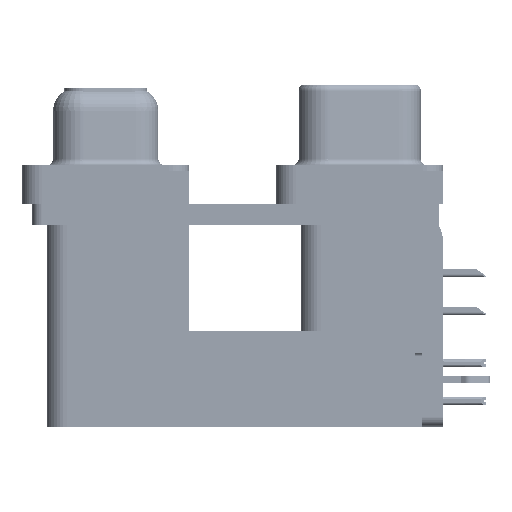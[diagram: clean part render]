
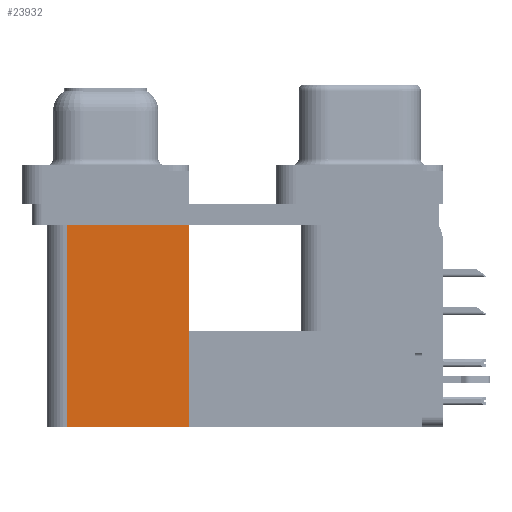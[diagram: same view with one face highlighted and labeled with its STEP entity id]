
A CAD part, left-side view. The second image highlights one B-rep face of the part: STEP entity #23932.
In plain terms, the highlighted planar face has unit normal (-1, 0, 0).
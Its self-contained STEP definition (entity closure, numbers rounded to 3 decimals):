
#1345 = CARTESIAN_POINT ( 'NONE',  ( 3.79, 21.975, -19.2 ) ) ;
#3859 = VERTEX_POINT ( 'NONE', #1345 ) ;
#4786 = DIRECTION ( 'NONE',  ( 0., 1., 0. ) ) ;
#5785 = DIRECTION ( 'NONE',  ( 0., 1., 0. ) ) ;
#5859 = EDGE_CURVE ( 'NONE', #43064, #3859, #52646, .T. ) ;
#6213 = ORIENTED_EDGE ( 'NONE', *, *, #5859, .F. ) ;
#8883 = VECTOR ( 'NONE', #54717, 1000. ) ;
#10048 = CARTESIAN_POINT ( 'NONE',  ( 3.79, 12.775, -2.5 ) ) ;
#10600 = VERTEX_POINT ( 'NONE', #32894 ) ;
#12820 = CARTESIAN_POINT ( 'NONE',  ( 3.79, 12.775, -19.2 ) ) ;
#14487 = ORIENTED_EDGE ( 'NONE', *, *, #58252, .F. ) ;
#14517 = EDGE_CURVE ( 'NONE', #10600, #62437, #56549, .T. ) ;
#16323 = DIRECTION ( 'NONE',  ( 1., 0., 0. ) ) ;
#16663 = FACE_OUTER_BOUND ( 'NONE', #61704, .T. ) ;
#20266 = CARTESIAN_POINT ( 'NONE',  ( 3.79, 21.975, -2.5 ) ) ;
#23932 = ADVANCED_FACE ( 'NONE', ( #16663 ), #64862, .F. ) ;
#25235 = CARTESIAN_POINT ( 'NONE',  ( 3.79, 12.775, -19.2 ) ) ;
#29400 = AXIS2_PLACEMENT_3D ( 'NONE', #42747, #16323, #48014 ) ;
#30411 = VECTOR ( 'NONE', #62018, 1000. ) ;
#32272 = ORIENTED_EDGE ( 'NONE', *, *, #59977, .T. ) ;
#32894 = CARTESIAN_POINT ( 'NONE',  ( 3.79, 12.775, -2.5 ) ) ;
#35319 = CARTESIAN_POINT ( 'NONE',  ( 3.79, 12.775, -19.2 ) ) ;
#35900 = VECTOR ( 'NONE', #4786, 1000. ) ;
#37487 = VECTOR ( 'NONE', #5785, 1000. ) ;
#40221 = LINE ( 'NONE', #35319, #30411 ) ;
#42747 = CARTESIAN_POINT ( 'NONE',  ( 3.79, 12.775, -19.2 ) ) ;
#43064 = VERTEX_POINT ( 'NONE', #12820 ) ;
#43125 = LINE ( 'NONE', #59322, #8883 ) ;
#48014 = DIRECTION ( 'NONE',  ( 0., 1., 0. ) ) ;
#52646 = LINE ( 'NONE', #25235, #35900 ) ;
#54717 = DIRECTION ( 'NONE',  ( 0., 0., 1. ) ) ;
#55279 = ORIENTED_EDGE ( 'NONE', *, *, #14517, .T. ) ;
#56549 = LINE ( 'NONE', #10048, #37487 ) ;
#58252 = EDGE_CURVE ( 'NONE', #3859, #62437, #43125, .T. ) ;
#59322 = CARTESIAN_POINT ( 'NONE',  ( 3.79, 21.975, -19.2 ) ) ;
#59977 = EDGE_CURVE ( 'NONE', #43064, #10600, #40221, .T. ) ;
#61704 = EDGE_LOOP ( 'NONE', ( #55279, #14487, #6213, #32272 ) ) ;
#62018 = DIRECTION ( 'NONE',  ( 0., 0., 1. ) ) ;
#62437 = VERTEX_POINT ( 'NONE', #20266 ) ;
#64862 = PLANE ( 'NONE',  #29400 ) ;
